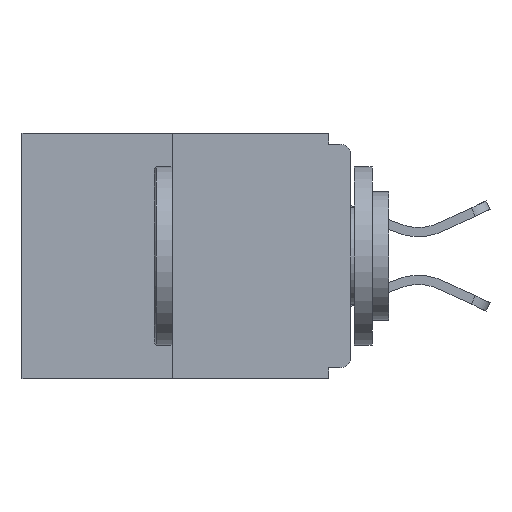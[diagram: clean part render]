
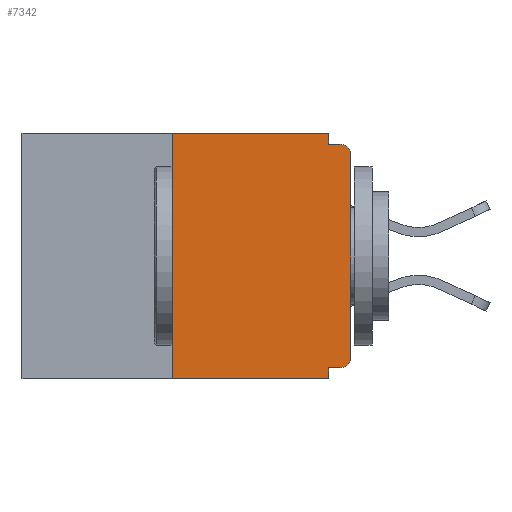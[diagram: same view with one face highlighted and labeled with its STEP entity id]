
A CAD part, left-side view. The second image highlights one B-rep face of the part: STEP entity #7342.
In plain terms, the highlighted planar face has unit normal (-1, 0, 0).
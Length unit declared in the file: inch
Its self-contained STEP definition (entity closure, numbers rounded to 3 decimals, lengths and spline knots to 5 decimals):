
#146 = DIRECTION ( 'NONE',  ( 0., 0., -1. ) ) ;
#208 = EDGE_CURVE ( 'NONE', #11470, #16358, #2270, .T. ) ;
#738 = CARTESIAN_POINT ( 'NONE',  ( 0., 0., -0.015 ) ) ;
#824 = VECTOR ( 'NONE', #8211, 39.37008 ) ;
#989 = ORIENTED_EDGE ( 'NONE', *, *, #6235, .T. ) ;
#2127 = CARTESIAN_POINT ( 'NONE',  ( 0., 0.46, 0. ) ) ;
#2270 = LINE ( 'NONE', #738, #21727 ) ;
#2345 = CARTESIAN_POINT ( 'NONE',  ( 0., 0.031, 0. ) ) ;
#2666 = DIRECTION ( 'NONE',  ( 0., 0., -1. ) ) ;
#2819 = VERTEX_POINT ( 'NONE', #10940 ) ;
#2831 = CARTESIAN_POINT ( 'NONE',  ( 0., 0.25, 0. ) ) ;
#2965 = CARTESIAN_POINT ( 'NONE',  ( 0., 0.46, -0.343 ) ) ;
#3256 = CARTESIAN_POINT ( 'NONE',  ( 0., 0.031, -0.328 ) ) ;
#3341 = CARTESIAN_POINT ( 'NONE',  ( 0., 0.015, -0.328 ) ) ;
#3515 = CARTESIAN_POINT ( 'NONE',  ( 0., 0.25, 0. ) ) ;
#4458 = VERTEX_POINT ( 'NONE', #10350 ) ;
#5437 = DIRECTION ( 'NONE',  ( 0., -1., 0. ) ) ;
#5725 = PLANE ( 'NONE',  #10029 ) ;
#5925 = VECTOR ( 'NONE', #8738, 39.37008 ) ;
#6189 = DIRECTION ( 'NONE',  ( -1., 0., 0. ) ) ;
#6235 = EDGE_CURVE ( 'NONE', #10963, #18594, #18399, .T. ) ;
#6410 = AXIS2_PLACEMENT_3D ( 'NONE', #15447, #6189, #22766 ) ;
#6763 = VERTEX_POINT ( 'NONE', #3256 ) ;
#7090 = CARTESIAN_POINT ( 'NONE',  ( 0., 0.031, -0.343 ) ) ;
#7211 = ORIENTED_EDGE ( 'NONE', *, *, #18962, .F. ) ;
#7342 = ADVANCED_FACE ( 'NONE', ( #16889 ), #5725, .F. ) ;
#7944 = CARTESIAN_POINT ( 'NONE',  ( 0., 0.015, -0.313 ) ) ;
#8004 = ORIENTED_EDGE ( 'NONE', *, *, #13070, .F. ) ;
#8211 = DIRECTION ( 'NONE',  ( 0., 0., 1. ) ) ;
#8226 = DIRECTION ( 'NONE',  ( 0., 1., 0. ) ) ;
#8431 = ORIENTED_EDGE ( 'NONE', *, *, #18495, .F. ) ;
#8738 = DIRECTION ( 'NONE',  ( 0., -1., 0. ) ) ;
#9414 = EDGE_CURVE ( 'NONE', #20342, #6763, #16555, .T. ) ;
#9754 = DIRECTION ( 'NONE',  ( 0., 0., -1. ) ) ;
#9890 = LINE ( 'NONE', #2965, #5925 ) ;
#10029 = AXIS2_PLACEMENT_3D ( 'NONE', #2127, #11095, #146 ) ;
#10350 = CARTESIAN_POINT ( 'NONE',  ( 0., 0.031, 0. ) ) ;
#10441 = ORIENTED_EDGE ( 'NONE', *, *, #13213, .T. ) ;
#10494 = CARTESIAN_POINT ( 'NONE',  ( 0., 0., 0. ) ) ;
#10506 = EDGE_CURVE ( 'NONE', #2819, #19157, #9890, .T. ) ;
#10640 = CARTESIAN_POINT ( 'NONE',  ( 0., 0.015, -0.015 ) ) ;
#10742 = CARTESIAN_POINT ( 'NONE',  ( 0., 0.46, 0. ) ) ;
#10829 = VECTOR ( 'NONE', #2666, 39.37008 ) ;
#10940 = CARTESIAN_POINT ( 'NONE',  ( 0., 0.25, -0.343 ) ) ;
#10963 = VERTEX_POINT ( 'NONE', #18948 ) ;
#11053 = VERTEX_POINT ( 'NONE', #3515 ) ;
#11095 = DIRECTION ( 'NONE',  ( 1., 0., 0. ) ) ;
#11470 = VERTEX_POINT ( 'NONE', #21522 ) ;
#11524 = LINE ( 'NONE', #2345, #22660 ) ;
#11686 = VECTOR ( 'NONE', #8226, 39.37008 ) ;
#11746 = ORIENTED_EDGE ( 'NONE', *, *, #21584, .F. ) ;
#12214 = CIRCLE ( 'NONE', #14569, 0.015 ) ;
#12949 = VECTOR ( 'NONE', #13872, 39.37008 ) ;
#13070 = EDGE_CURVE ( 'NONE', #11053, #4458, #16213, .T. ) ;
#13213 = EDGE_CURVE ( 'NONE', #20342, #10963, #12214, .T. ) ;
#13872 = DIRECTION ( 'NONE',  ( 0., 0., 1. ) ) ;
#14569 = AXIS2_PLACEMENT_3D ( 'NONE', #7944, #20703, #9754 ) ;
#15447 = CARTESIAN_POINT ( 'NONE',  ( 0., 0.015, -0.03 ) ) ;
#15926 = VECTOR ( 'NONE', #5437, 39.37008 ) ;
#16213 = LINE ( 'NONE', #10742, #15926 ) ;
#16358 = VERTEX_POINT ( 'NONE', #10640 ) ;
#16555 = LINE ( 'NONE', #17251, #11686 ) ;
#16836 = ORIENTED_EDGE ( 'NONE', *, *, #208, .F. ) ;
#16889 = FACE_OUTER_BOUND ( 'NONE', #18242, .T. ) ;
#16991 = DIRECTION ( 'NONE',  ( 0., 0., -1. ) ) ;
#17070 = CARTESIAN_POINT ( 'NONE',  ( 0., 0.031, -0.343 ) ) ;
#17226 = DIRECTION ( 'NONE',  ( 0., -1., 0. ) ) ;
#17251 = CARTESIAN_POINT ( 'NONE',  ( 0., 0., -0.328 ) ) ;
#17395 = CARTESIAN_POINT ( 'NONE',  ( 0., 0., -0.03 ) ) ;
#18242 = EDGE_LOOP ( 'NONE', ( #8004, #7211, #20968, #8431, #19857, #10441, #989, #22575, #16836, #11746 ) ) ;
#18399 = LINE ( 'NONE', #10494, #12949 ) ;
#18495 = EDGE_CURVE ( 'NONE', #6763, #19157, #18563, .T. ) ;
#18563 = LINE ( 'NONE', #17070, #10829 ) ;
#18594 = VERTEX_POINT ( 'NONE', #17395 ) ;
#18948 = CARTESIAN_POINT ( 'NONE',  ( 0., 0., -0.313 ) ) ;
#18962 = EDGE_CURVE ( 'NONE', #2819, #11053, #22286, .T. ) ;
#19157 = VERTEX_POINT ( 'NONE', #7090 ) ;
#19857 = ORIENTED_EDGE ( 'NONE', *, *, #9414, .F. ) ;
#20117 = EDGE_CURVE ( 'NONE', #18594, #16358, #21300, .T. ) ;
#20342 = VERTEX_POINT ( 'NONE', #3341 ) ;
#20703 = DIRECTION ( 'NONE',  ( -1., 0., 0. ) ) ;
#20968 = ORIENTED_EDGE ( 'NONE', *, *, #10506, .T. ) ;
#21300 = CIRCLE ( 'NONE', #6410, 0.015 ) ;
#21522 = CARTESIAN_POINT ( 'NONE',  ( 0., 0.031, -0.015 ) ) ;
#21584 = EDGE_CURVE ( 'NONE', #4458, #11470, #11524, .T. ) ;
#21727 = VECTOR ( 'NONE', #17226, 39.37008 ) ;
#22286 = LINE ( 'NONE', #2831, #824 ) ;
#22575 = ORIENTED_EDGE ( 'NONE', *, *, #20117, .T. ) ;
#22660 = VECTOR ( 'NONE', #16991, 39.37008 ) ;
#22766 = DIRECTION ( 'NONE',  ( 0., 0., -1. ) ) ;
